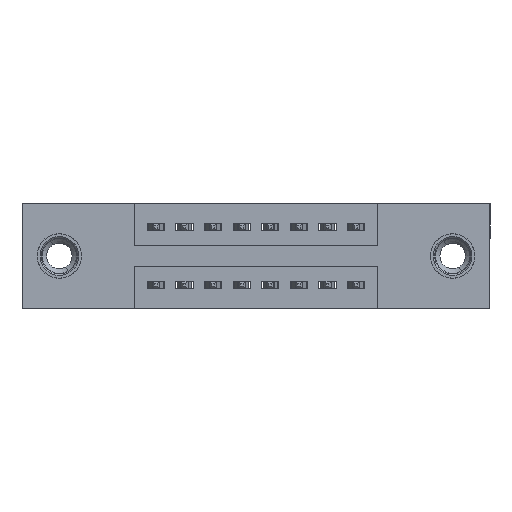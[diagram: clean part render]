
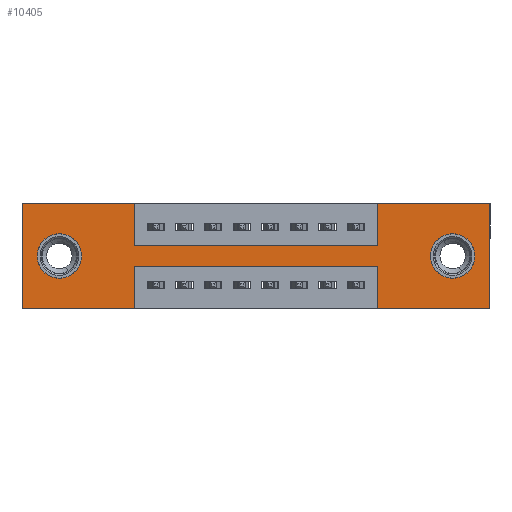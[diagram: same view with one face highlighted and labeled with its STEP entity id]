
A CAD part, front view. The second image highlights one B-rep face of the part: STEP entity #10405.
In plain terms, the highlighted planar face has unit normal (0, -1, 0).
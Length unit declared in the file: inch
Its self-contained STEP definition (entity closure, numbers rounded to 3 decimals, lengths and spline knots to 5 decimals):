
#570 = DIRECTION ( 'NONE',  ( 0., -1., 0. ) ) ;
#777 = VECTOR ( 'NONE', #14487, 39.37008 ) ;
#778 = DIRECTION ( 'NONE',  ( 0., 1., 0. ) ) ;
#863 = ORIENTED_EDGE ( 'NONE', *, *, #12828, .F. ) ;
#1207 = VERTEX_POINT ( 'NONE', #13507 ) ;
#1362 = LINE ( 'NONE', #7612, #13258 ) ;
#1412 = EDGE_LOOP ( 'NONE', ( #11312, #10563 ) ) ;
#1421 = AXIS2_PLACEMENT_3D ( 'NONE', #9032, #570, #12853 ) ;
#1590 = CARTESIAN_POINT ( 'NONE',  ( 0.13, 0., -0.263 ) ) ;
#1668 = VECTOR ( 'NONE', #8510, 39.37008 ) ;
#1707 = VERTEX_POINT ( 'NONE', #9780 ) ;
#1906 = CARTESIAN_POINT ( 'NONE',  ( 0., 0., 0. ) ) ;
#1962 = AXIS2_PLACEMENT_3D ( 'NONE', #6642, #7641, #13811 ) ;
#2288 = ORIENTED_EDGE ( 'NONE', *, *, #10717, .F. ) ;
#2308 = CARTESIAN_POINT ( 'NONE',  ( 1.635, 0., -0.37 ) ) ;
#2423 = CARTESIAN_POINT ( 'NONE',  ( 1.635, 0., 0. ) ) ;
#2505 = CARTESIAN_POINT ( 'NONE',  ( 0., 0., 0. ) ) ;
#2515 = VERTEX_POINT ( 'NONE', #11258 ) ;
#2708 = LINE ( 'NONE', #2505, #4566 ) ;
#2724 = CIRCLE ( 'NONE', #7234, 0.078 ) ;
#2825 = LINE ( 'NONE', #13643, #8840 ) ;
#3053 = VECTOR ( 'NONE', #11574, 39.37008 ) ;
#3108 = PLANE ( 'NONE',  #1421 ) ;
#3155 = VECTOR ( 'NONE', #10899, 39.37008 ) ;
#3231 = ORIENTED_EDGE ( 'NONE', *, *, #10172, .T. ) ;
#3469 = VERTEX_POINT ( 'NONE', #7221 ) ;
#3520 = LINE ( 'NONE', #2423, #3155 ) ;
#3600 = CARTESIAN_POINT ( 'NONE',  ( 0.3925, 0., -0.15 ) ) ;
#3748 = VERTEX_POINT ( 'NONE', #10996 ) ;
#3820 = CARTESIAN_POINT ( 'NONE',  ( 0.3925, 0., 0. ) ) ;
#3895 = VERTEX_POINT ( 'NONE', #14247 ) ;
#3939 = LINE ( 'NONE', #8669, #1668 ) ;
#3949 = VERTEX_POINT ( 'NONE', #11904 ) ;
#4377 = EDGE_CURVE ( 'NONE', #1707, #11511, #12406, .T. ) ;
#4392 = EDGE_CURVE ( 'NONE', #3895, #6069, #13549, .T. ) ;
#4465 = DIRECTION ( 'NONE',  ( 0., 0., 1. ) ) ;
#4487 = CARTESIAN_POINT ( 'NONE',  ( 0., 0., 0. ) ) ;
#4566 = VECTOR ( 'NONE', #4887, 39.37008 ) ;
#4645 = ORIENTED_EDGE ( 'NONE', *, *, #10377, .F. ) ;
#4666 = VECTOR ( 'NONE', #14974, 39.37008 ) ;
#4688 = CARTESIAN_POINT ( 'NONE',  ( 0., 0., -0.37 ) ) ;
#4824 = EDGE_CURVE ( 'NONE', #3949, #3469, #14494, .T. ) ;
#4851 = LINE ( 'NONE', #3820, #13570 ) ;
#4867 = FACE_OUTER_BOUND ( 'NONE', #7108, .T. ) ;
#4887 = DIRECTION ( 'NONE',  ( 1., 0., 0. ) ) ;
#5266 = AXIS2_PLACEMENT_3D ( 'NONE', #5367, #13955, #10129 ) ;
#5284 = LINE ( 'NONE', #4688, #777 ) ;
#5367 = CARTESIAN_POINT ( 'NONE',  ( 0.13, 0., -0.185 ) ) ;
#5450 = CARTESIAN_POINT ( 'NONE',  ( 0.3925, 0., -0.37 ) ) ;
#5644 = VERTEX_POINT ( 'NONE', #9391 ) ;
#6069 = VERTEX_POINT ( 'NONE', #1590 ) ;
#6642 = CARTESIAN_POINT ( 'NONE',  ( 1.505, 0., -0.185 ) ) ;
#6777 = LINE ( 'NONE', #12702, #3053 ) ;
#6829 = CARTESIAN_POINT ( 'NONE',  ( 0., 0., -0.37 ) ) ;
#6919 = ORIENTED_EDGE ( 'NONE', *, *, #11153, .F. ) ;
#6935 = ORIENTED_EDGE ( 'NONE', *, *, #10015, .F. ) ;
#7006 = ORIENTED_EDGE ( 'NONE', *, *, #4392, .T. ) ;
#7107 = VECTOR ( 'NONE', #4465, 39.37008 ) ;
#7108 = EDGE_LOOP ( 'NONE', ( #8109, #2288, #15228, #11065, #8329, #9159, #6935, #10399, #6919, #9381, #863, #4645 ) ) ;
#7221 = CARTESIAN_POINT ( 'NONE',  ( 0.3925, 0., -0.37 ) ) ;
#7234 = AXIS2_PLACEMENT_3D ( 'NONE', #9335, #778, #10590 ) ;
#7612 = CARTESIAN_POINT ( 'NONE',  ( 0., 0., 0. ) ) ;
#7630 = EDGE_CURVE ( 'NONE', #11511, #1707, #2724, .T. ) ;
#7641 = DIRECTION ( 'NONE',  ( 0., 1., 0. ) ) ;
#7733 = DIRECTION ( 'NONE',  ( 0., 0., -1. ) ) ;
#8109 = ORIENTED_EDGE ( 'NONE', *, *, #4824, .F. ) ;
#8329 = ORIENTED_EDGE ( 'NONE', *, *, #14561, .F. ) ;
#8349 = EDGE_CURVE ( 'NONE', #11597, #9928, #2708, .T. ) ;
#8462 = CARTESIAN_POINT ( 'NONE',  ( 0.13, 0., -0.185 ) ) ;
#8510 = DIRECTION ( 'NONE',  ( -1., 0., 0. ) ) ;
#8582 = DIRECTION ( 'NONE',  ( 0., 0., 1. ) ) ;
#8669 = CARTESIAN_POINT ( 'NONE',  ( 0., 0., -0.37 ) ) ;
#8679 = DIRECTION ( 'NONE',  ( 1., 0., 0. ) ) ;
#8748 = EDGE_CURVE ( 'NONE', #10065, #2515, #1362, .T. ) ;
#8840 = VECTOR ( 'NONE', #11236, 39.37008 ) ;
#9032 = CARTESIAN_POINT ( 'NONE',  ( 0., 0., -0.37 ) ) ;
#9159 = ORIENTED_EDGE ( 'NONE', *, *, #8349, .F. ) ;
#9335 = CARTESIAN_POINT ( 'NONE',  ( 1.505, 0., -0.185 ) ) ;
#9381 = ORIENTED_EDGE ( 'NONE', *, *, #8748, .F. ) ;
#9391 = CARTESIAN_POINT ( 'NONE',  ( 1.2425, 0., -0.22 ) ) ;
#9752 = LINE ( 'NONE', #1906, #7107 ) ;
#9780 = CARTESIAN_POINT ( 'NONE',  ( 1.505, 0., -0.107 ) ) ;
#9928 = VERTEX_POINT ( 'NONE', #14762 ) ;
#9956 = EDGE_LOOP ( 'NONE', ( #7006, #3231 ) ) ;
#9992 = EDGE_CURVE ( 'NONE', #1207, #5644, #6777, .T. ) ;
#10015 = EDGE_CURVE ( 'NONE', #3748, #11597, #13808, .T. ) ;
#10025 = CARTESIAN_POINT ( 'NONE',  ( 0.3925, 0., -0.15 ) ) ;
#10065 = VERTEX_POINT ( 'NONE', #4487 ) ;
#10129 = DIRECTION ( 'NONE',  ( 0., 0., 1. ) ) ;
#10172 = EDGE_CURVE ( 'NONE', #6069, #3895, #12668, .T. ) ;
#10377 = EDGE_CURVE ( 'NONE', #3469, #14413, #5284, .T. ) ;
#10399 = ORIENTED_EDGE ( 'NONE', *, *, #10655, .F. ) ;
#10405 = ADVANCED_FACE ( 'NONE', ( #12076, #12461, #4867 ), #3108, .T. ) ;
#10563 = ORIENTED_EDGE ( 'NONE', *, *, #7630, .T. ) ;
#10590 = DIRECTION ( 'NONE',  ( 0., 0., -1. ) ) ;
#10655 = EDGE_CURVE ( 'NONE', #15387, #3748, #13586, .T. ) ;
#10717 = EDGE_CURVE ( 'NONE', #5644, #3949, #2825, .T. ) ;
#10899 = DIRECTION ( 'NONE',  ( 0., 0., -1. ) ) ;
#10996 = CARTESIAN_POINT ( 'NONE',  ( 1.2425, 0., -0.15 ) ) ;
#11065 = ORIENTED_EDGE ( 'NONE', *, *, #11343, .F. ) ;
#11153 = EDGE_CURVE ( 'NONE', #2515, #15387, #4851, .T. ) ;
#11236 = DIRECTION ( 'NONE',  ( -1., 0., 0. ) ) ;
#11258 = CARTESIAN_POINT ( 'NONE',  ( 0.3925, 0., 0. ) ) ;
#11286 = VECTOR ( 'NONE', #7733, 39.37008 ) ;
#11312 = ORIENTED_EDGE ( 'NONE', *, *, #4377, .T. ) ;
#11343 = EDGE_CURVE ( 'NONE', #14664, #1207, #3939, .T. ) ;
#11511 = VERTEX_POINT ( 'NONE', #14304 ) ;
#11574 = DIRECTION ( 'NONE',  ( 0., 0., 1. ) ) ;
#11597 = VERTEX_POINT ( 'NONE', #13353 ) ;
#11904 = CARTESIAN_POINT ( 'NONE',  ( 0.3925, 0., -0.22 ) ) ;
#12076 = FACE_BOUND ( 'NONE', #1412, .T. ) ;
#12249 = DIRECTION ( 'NONE',  ( 0., 0., -1. ) ) ;
#12406 = CIRCLE ( 'NONE', #1962, 0.078 ) ;
#12461 = FACE_BOUND ( 'NONE', #9956, .T. ) ;
#12668 = CIRCLE ( 'NONE', #14877, 0.078 ) ;
#12702 = CARTESIAN_POINT ( 'NONE',  ( 1.2425, 0., -0.37 ) ) ;
#12806 = DIRECTION ( 'NONE',  ( 0., 0., 1. ) ) ;
#12828 = EDGE_CURVE ( 'NONE', #14413, #10065, #9752, .T. ) ;
#12853 = DIRECTION ( 'NONE',  ( 0., 0., -1. ) ) ;
#13189 = DIRECTION ( 'NONE',  ( 0., 1., 0. ) ) ;
#13258 = VECTOR ( 'NONE', #8679, 39.37008 ) ;
#13353 = CARTESIAN_POINT ( 'NONE',  ( 1.2425, 0., 0. ) ) ;
#13421 = VECTOR ( 'NONE', #12806, 39.37008 ) ;
#13507 = CARTESIAN_POINT ( 'NONE',  ( 1.2425, 0., -0.37 ) ) ;
#13549 = CIRCLE ( 'NONE', #5266, 0.078 ) ;
#13570 = VECTOR ( 'NONE', #12249, 39.37008 ) ;
#13586 = LINE ( 'NONE', #10025, #4666 ) ;
#13643 = CARTESIAN_POINT ( 'NONE',  ( 0.3925, 0., -0.22 ) ) ;
#13808 = LINE ( 'NONE', #14020, #13421 ) ;
#13811 = DIRECTION ( 'NONE',  ( 0., 0., -1. ) ) ;
#13955 = DIRECTION ( 'NONE',  ( 0., 1., 0. ) ) ;
#14020 = CARTESIAN_POINT ( 'NONE',  ( 1.2425, 0., 0. ) ) ;
#14247 = CARTESIAN_POINT ( 'NONE',  ( 0.13, 0., -0.107 ) ) ;
#14304 = CARTESIAN_POINT ( 'NONE',  ( 1.505, 0., -0.263 ) ) ;
#14413 = VERTEX_POINT ( 'NONE', #6829 ) ;
#14487 = DIRECTION ( 'NONE',  ( -1., 0., 0. ) ) ;
#14494 = LINE ( 'NONE', #5450, #11286 ) ;
#14561 = EDGE_CURVE ( 'NONE', #9928, #14664, #3520, .T. ) ;
#14664 = VERTEX_POINT ( 'NONE', #2308 ) ;
#14762 = CARTESIAN_POINT ( 'NONE',  ( 1.635, 0., 0. ) ) ;
#14877 = AXIS2_PLACEMENT_3D ( 'NONE', #8462, #13189, #8582 ) ;
#14974 = DIRECTION ( 'NONE',  ( 1., 0., 0. ) ) ;
#15228 = ORIENTED_EDGE ( 'NONE', *, *, #9992, .F. ) ;
#15387 = VERTEX_POINT ( 'NONE', #3600 ) ;
